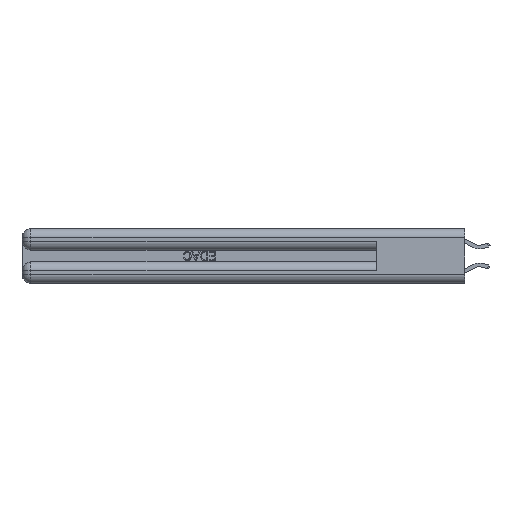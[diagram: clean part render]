
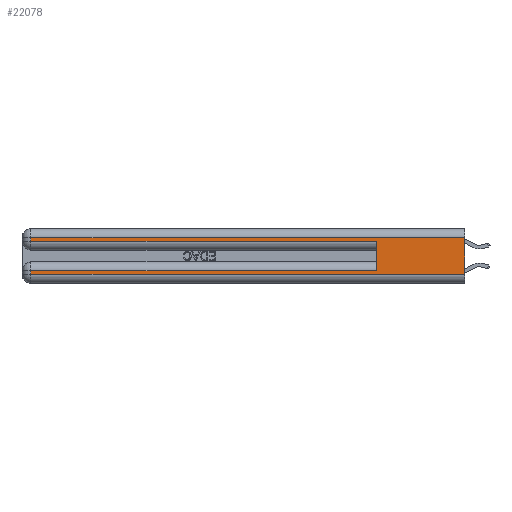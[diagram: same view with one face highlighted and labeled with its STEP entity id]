
A CAD part, left-side view. The second image highlights one B-rep face of the part: STEP entity #22078.
In plain terms, the highlighted planar face has unit normal (-1, 0, 0).
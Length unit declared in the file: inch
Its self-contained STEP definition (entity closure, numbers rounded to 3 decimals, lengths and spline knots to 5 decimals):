
#2 = AXIS2_PLACEMENT_3D ( 'NONE', #13174, #5740, #31310 ) ;
#1386 = CARTESIAN_POINT ( 'NONE',  ( 0., 0., 0.06 ) ) ;
#2511 = LINE ( 'NONE', #4142, #22305 ) ;
#2557 = DIRECTION ( 'NONE',  ( 0., 1., 0. ) ) ;
#2583 = ORIENTED_EDGE ( 'NONE', *, *, #11645, .T. ) ;
#3186 = EDGE_CURVE ( 'NONE', #4114, #33164, #6634, .T. ) ;
#4037 = CARTESIAN_POINT ( 'NONE',  ( 0., 0., 0.06 ) ) ;
#4114 = VERTEX_POINT ( 'NONE', #20271 ) ;
#4142 = CARTESIAN_POINT ( 'NONE',  ( 0., 2.94, 0.37 ) ) ;
#4648 = LINE ( 'NONE', #31299, #7478 ) ;
#4784 = LINE ( 'NONE', #33169, #8804 ) ;
#5520 = FACE_OUTER_BOUND ( 'NONE', #25389, .T. ) ;
#5734 = DIRECTION ( 'NONE',  ( 0., 0., -1. ) ) ;
#5740 = DIRECTION ( 'NONE',  ( 1., 0., 0. ) ) ;
#5977 = LINE ( 'NONE', #23169, #22147 ) ;
#6634 = LINE ( 'NONE', #21668, #23181 ) ;
#7139 = EDGE_CURVE ( 'NONE', #8980, #10682, #4784, .T. ) ;
#7478 = VECTOR ( 'NONE', #5734, 39.37008 ) ;
#8683 = DIRECTION ( 'NONE',  ( 0., -1., 0. ) ) ;
#8804 = VECTOR ( 'NONE', #2557, 39.37008 ) ;
#8907 = VERTEX_POINT ( 'NONE', #4037 ) ;
#8980 = VERTEX_POINT ( 'NONE', #29676 ) ;
#9717 = CARTESIAN_POINT ( 'NONE',  ( 0., 2.94, 0.31 ) ) ;
#10682 = VERTEX_POINT ( 'NONE', #9717 ) ;
#10727 = VERTEX_POINT ( 'NONE', #18108 ) ;
#11329 = EDGE_CURVE ( 'NONE', #10727, #8907, #23536, .T. ) ;
#11645 = EDGE_CURVE ( 'NONE', #33164, #10727, #2511, .T. ) ;
#12053 = ORIENTED_EDGE ( 'NONE', *, *, #7139, .T. ) ;
#12938 = VECTOR ( 'NONE', #8683, 39.37008 ) ;
#13174 = CARTESIAN_POINT ( 'NONE',  ( 0., 0., 0.37 ) ) ;
#13983 = EDGE_CURVE ( 'NONE', #8980, #8907, #4648, .T. ) ;
#16396 = CARTESIAN_POINT ( 'NONE',  ( 0., 0.6, 0.145 ) ) ;
#17963 = LINE ( 'NONE', #16396, #27637 ) ;
#18108 = CARTESIAN_POINT ( 'NONE',  ( 0., 2.94, 0.06 ) ) ;
#18628 = ORIENTED_EDGE ( 'NONE', *, *, #3186, .T. ) ;
#18710 = ORIENTED_EDGE ( 'NONE', *, *, #11329, .T. ) ;
#18762 = CARTESIAN_POINT ( 'NONE',  ( 0., 0.6, 0.285 ) ) ;
#19136 = DIRECTION ( 'NONE',  ( 0., 0., 1. ) ) ;
#19458 = ORIENTED_EDGE ( 'NONE', *, *, #21372, .T. ) ;
#20271 = CARTESIAN_POINT ( 'NONE',  ( 0., 0.6, 0.085 ) ) ;
#20819 = VERTEX_POINT ( 'NONE', #25165 ) ;
#21372 = EDGE_CURVE ( 'NONE', #10682, #20819, #5977, .T. ) ;
#21458 = DIRECTION ( 'NONE',  ( 0., 1., 0. ) ) ;
#21668 = CARTESIAN_POINT ( 'NONE',  ( 0., 0., 0.085 ) ) ;
#21686 = CARTESIAN_POINT ( 'NONE',  ( 0., 2.94, 0.085 ) ) ;
#22078 = ADVANCED_FACE ( 'NONE', ( #5520 ), #26148, .F. ) ;
#22147 = VECTOR ( 'NONE', #25959, 39.37008 ) ;
#22305 = VECTOR ( 'NONE', #27579, 39.37008 ) ;
#22911 = ORIENTED_EDGE ( 'NONE', *, *, #32616, .F. ) ;
#23169 = CARTESIAN_POINT ( 'NONE',  ( 0., 2.94, 0.37 ) ) ;
#23181 = VECTOR ( 'NONE', #21458, 39.37008 ) ;
#23536 = LINE ( 'NONE', #1386, #23929 ) ;
#23929 = VECTOR ( 'NONE', #24733, 39.37008 ) ;
#24733 = DIRECTION ( 'NONE',  ( 0., -1., 0. ) ) ;
#25165 = CARTESIAN_POINT ( 'NONE',  ( 0., 2.94, 0.285 ) ) ;
#25389 = EDGE_LOOP ( 'NONE', ( #29829, #12053, #19458, #30988, #22911, #18628, #2583, #18710 ) ) ;
#25959 = DIRECTION ( 'NONE',  ( 0., 0., -1. ) ) ;
#26148 = PLANE ( 'NONE',  #2 ) ;
#27579 = DIRECTION ( 'NONE',  ( 0., 0., -1. ) ) ;
#27637 = VECTOR ( 'NONE', #19136, 39.37008 ) ;
#28021 = VERTEX_POINT ( 'NONE', #18762 ) ;
#28141 = EDGE_CURVE ( 'NONE', #20819, #28021, #32659, .T. ) ;
#29440 = CARTESIAN_POINT ( 'NONE',  ( 0., 0., 0.285 ) ) ;
#29676 = CARTESIAN_POINT ( 'NONE',  ( 0., 0., 0.31 ) ) ;
#29829 = ORIENTED_EDGE ( 'NONE', *, *, #13983, .F. ) ;
#30988 = ORIENTED_EDGE ( 'NONE', *, *, #28141, .T. ) ;
#31299 = CARTESIAN_POINT ( 'NONE',  ( 0., 0., 0.37 ) ) ;
#31310 = DIRECTION ( 'NONE',  ( 0., 0., -1. ) ) ;
#32616 = EDGE_CURVE ( 'NONE', #4114, #28021, #17963, .T. ) ;
#32659 = LINE ( 'NONE', #29440, #12938 ) ;
#33164 = VERTEX_POINT ( 'NONE', #21686 ) ;
#33169 = CARTESIAN_POINT ( 'NONE',  ( 0., 0., 0.31 ) ) ;
